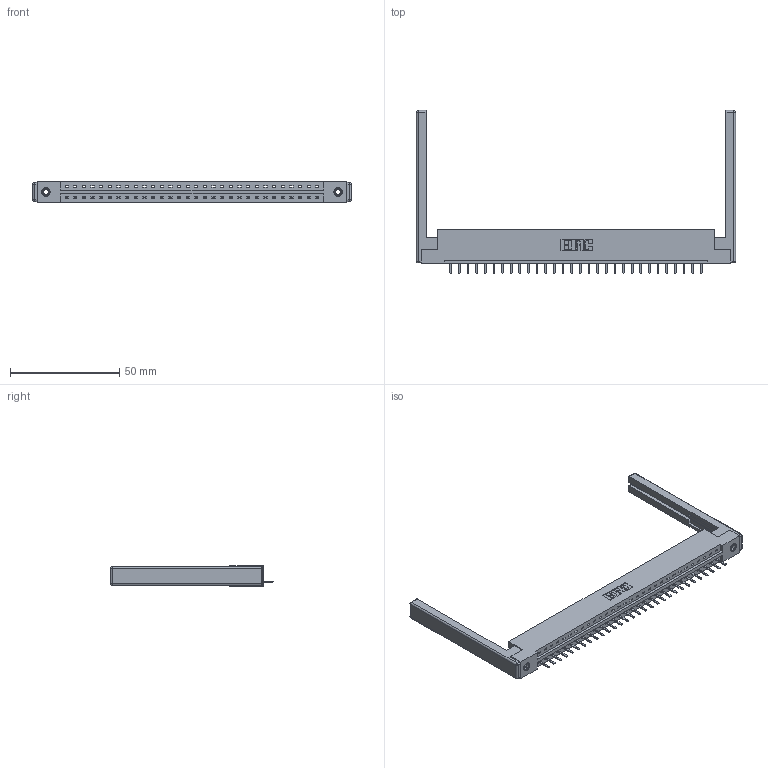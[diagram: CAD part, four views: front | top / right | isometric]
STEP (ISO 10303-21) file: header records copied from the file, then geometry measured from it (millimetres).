
FILE_DESCRIPTION (( 'STEP AP203' ), '1' );
FILE_NAME ('387-030-520-168.STEP', '2019-10-03T17:43:47', ( '' ), ( '' ), 'SwSTEP 2.0', 'SolidWorks 2016', '' );
FILE_SCHEMA (( 'CONFIG_CONTROL_DESIGN' ));
Length unit declared in the file: inch
Products named in the file (5): 387-030-520-168; 345-250-001_345-250-001-102; 345-292-001_345-293-120; 307-220-068; 337 Part_Flush Mounting Lugs - 0.156 Dia-TI
Assembly tree (35 placements, depth 2):
  387-030-520-168
    337 Part_Flush Mounting Lugs - 0.156 Dia-TI
    345-292-001_345-293-120  x30
    345-250-001_345-250-001-102  x2
    307-220-068  x2
Bounding box: 146.3 x 74.76 x 9.4 mm (x, y, z)
Volume: 19360.6 mm3; surface area: 19184.1 mm2
Topology: 35 solids, 35 shells, 2248 faces, 6581 edges, 4286 vertices
Faces by surface type: plane 1598, cylinder 626, cone 12, sphere 8, torus 4
Entity records: 26726 total; most frequent: CARTESIAN_POINT 4621, ORIENTED_EDGE 4564, DIRECTION 3976, EDGE_CURVE 2282, LINE 2100, VECTOR 2100, VERTEX_POINT 1510, AXIS2_PLACEMENT_3D 938
